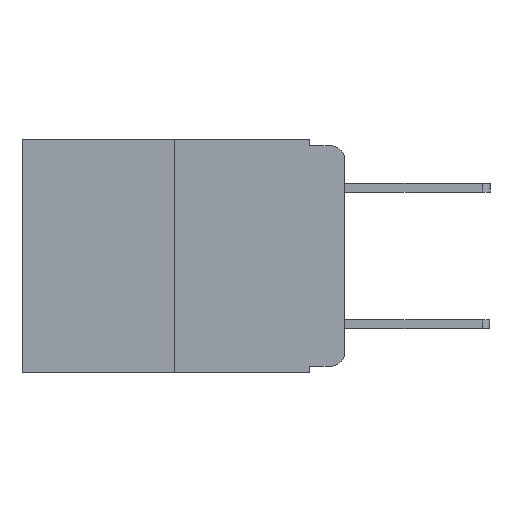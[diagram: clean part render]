
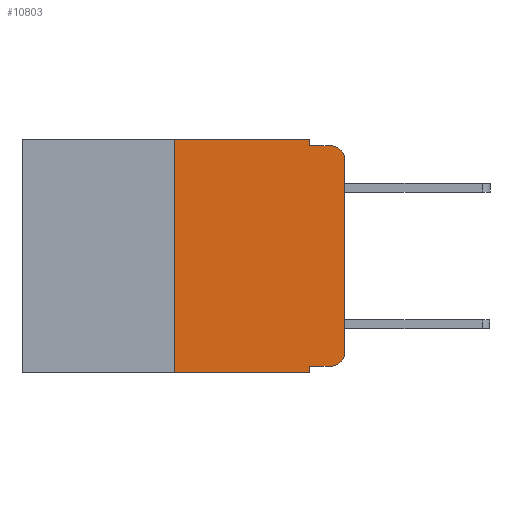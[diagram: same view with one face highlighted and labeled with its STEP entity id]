
A CAD part, left-side view. The second image highlights one B-rep face of the part: STEP entity #10803.
In plain terms, the highlighted planar face has unit normal (-1, 0, 0).
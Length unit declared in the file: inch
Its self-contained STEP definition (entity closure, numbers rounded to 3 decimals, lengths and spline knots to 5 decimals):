
#168 = LINE ( 'NONE', #14847, #4558 ) ;
#175 = LINE ( 'NONE', #13867, #18776 ) ;
#772 = ORIENTED_EDGE ( 'NONE', *, *, #3766, .T. ) ;
#1651 = ORIENTED_EDGE ( 'NONE', *, *, #4543, .F. ) ;
#1679 = VECTOR ( 'NONE', #12009, 39.37008 ) ;
#2320 = LINE ( 'NONE', #2339, #20710 ) ;
#2339 = CARTESIAN_POINT ( 'NONE',  ( 0., 0., 0. ) ) ;
#2484 = CARTESIAN_POINT ( 'NONE',  ( 0., 0.051, -0.333 ) ) ;
#2828 = EDGE_CURVE ( 'NONE', #6798, #6359, #2320, .T. ) ;
#2835 = CARTESIAN_POINT ( 'NONE',  ( 0., 0.02, -0.333 ) ) ;
#2984 = VERTEX_POINT ( 'NONE', #10625 ) ;
#3086 = VERTEX_POINT ( 'NONE', #10299 ) ;
#3766 = EDGE_CURVE ( 'NONE', #23074, #15496, #11955, .T. ) ;
#4369 = FACE_OUTER_BOUND ( 'NONE', #20748, .T. ) ;
#4543 = EDGE_CURVE ( 'NONE', #9731, #9596, #175, .T. ) ;
#4558 = VECTOR ( 'NONE', #9548, 39.37008 ) ;
#4666 = VECTOR ( 'NONE', #14319, 39.37008 ) ;
#4750 = AXIS2_PLACEMENT_3D ( 'NONE', #20246, #9752, #21972 ) ;
#4776 = LINE ( 'NONE', #7877, #17878 ) ;
#5048 = CARTESIAN_POINT ( 'NONE',  ( 0., 0.473, 0. ) ) ;
#5425 = ORIENTED_EDGE ( 'NONE', *, *, #19285, .F. ) ;
#5582 = CARTESIAN_POINT ( 'NONE',  ( 0., 0.25, 0. ) ) ;
#5977 = CARTESIAN_POINT ( 'NONE',  ( 0., 0.051, 0. ) ) ;
#6223 = EDGE_CURVE ( 'NONE', #23074, #15242, #4776, .T. ) ;
#6258 = EDGE_CURVE ( 'NONE', #2984, #15242, #22451, .T. ) ;
#6303 = ORIENTED_EDGE ( 'NONE', *, *, #10208, .T. ) ;
#6359 = VERTEX_POINT ( 'NONE', #14167 ) ;
#6413 = DIRECTION ( 'NONE',  ( 0., 0., -1. ) ) ;
#6798 = VERTEX_POINT ( 'NONE', #8709 ) ;
#6996 = EDGE_CURVE ( 'NONE', #3086, #23016, #12933, .T. ) ;
#7148 = AXIS2_PLACEMENT_3D ( 'NONE', #20542, #10077, #22284 ) ;
#7418 = ORIENTED_EDGE ( 'NONE', *, *, #2828, .T. ) ;
#7732 = DIRECTION ( 'NONE',  ( 0., -1., 0. ) ) ;
#7877 = CARTESIAN_POINT ( 'NONE',  ( 0., 0.051, 0. ) ) ;
#7896 = VECTOR ( 'NONE', #22745, 39.37008 ) ;
#8709 = CARTESIAN_POINT ( 'NONE',  ( 0., 0., -0.313 ) ) ;
#9112 = ORIENTED_EDGE ( 'NONE', *, *, #6996, .F. ) ;
#9129 = CARTESIAN_POINT ( 'NONE',  ( 0., 0.473, -0.343 ) ) ;
#9548 = DIRECTION ( 'NONE',  ( 0., 0., 1. ) ) ;
#9596 = VERTEX_POINT ( 'NONE', #5977 ) ;
#9731 = VERTEX_POINT ( 'NONE', #5582 ) ;
#9752 = DIRECTION ( 'NONE',  ( -1., 0., 0. ) ) ;
#10077 = DIRECTION ( 'NONE',  ( -1., 0., 0. ) ) ;
#10208 = EDGE_CURVE ( 'NONE', #15496, #6798, #22122, .T. ) ;
#10299 = CARTESIAN_POINT ( 'NONE',  ( 0., 0.051, -0.01 ) ) ;
#10394 = DIRECTION ( 'NONE',  ( 0., 0., 1. ) ) ;
#10507 = DIRECTION ( 'NONE',  ( 0., 0., -1. ) ) ;
#10625 = CARTESIAN_POINT ( 'NONE',  ( 0., 0.25, -0.343 ) ) ;
#10803 = ADVANCED_FACE ( 'NONE', ( #4369 ), #22634, .F. ) ;
#11955 = LINE ( 'NONE', #11986, #1679 ) ;
#11986 = CARTESIAN_POINT ( 'NONE',  ( 0., 0.051, -0.333 ) ) ;
#12009 = DIRECTION ( 'NONE',  ( 0., -1., 0. ) ) ;
#12540 = CARTESIAN_POINT ( 'NONE',  ( 0., 0.051, 0. ) ) ;
#12930 = CARTESIAN_POINT ( 'NONE',  ( 0., 0.051, -0.343 ) ) ;
#12933 = LINE ( 'NONE', #19776, #21065 ) ;
#13134 = LINE ( 'NONE', #12540, #4666 ) ;
#13308 = ORIENTED_EDGE ( 'NONE', *, *, #14182, .T. ) ;
#13439 = EDGE_CURVE ( 'NONE', #2984, #9731, #168, .T. ) ;
#13588 = ORIENTED_EDGE ( 'NONE', *, *, #6223, .F. ) ;
#13867 = CARTESIAN_POINT ( 'NONE',  ( 0., 0.473, 0. ) ) ;
#14167 = CARTESIAN_POINT ( 'NONE',  ( 0., 0., -0.03 ) ) ;
#14182 = EDGE_CURVE ( 'NONE', #6359, #23016, #14995, .T. ) ;
#14319 = DIRECTION ( 'NONE',  ( 0., 0., -1. ) ) ;
#14847 = CARTESIAN_POINT ( 'NONE',  ( 0., 0.25, 0. ) ) ;
#14995 = CIRCLE ( 'NONE', #4750, 0.02 ) ;
#15242 = VERTEX_POINT ( 'NONE', #12930 ) ;
#15496 = VERTEX_POINT ( 'NONE', #2835 ) ;
#15664 = AXIS2_PLACEMENT_3D ( 'NONE', #5048, #20970, #10507 ) ;
#16391 = DIRECTION ( 'NONE',  ( 0., -1., 0. ) ) ;
#16599 = ORIENTED_EDGE ( 'NONE', *, *, #13439, .F. ) ;
#17878 = VECTOR ( 'NONE', #6413, 39.37008 ) ;
#18776 = VECTOR ( 'NONE', #7732, 39.37008 ) ;
#19285 = EDGE_CURVE ( 'NONE', #9596, #3086, #13134, .T. ) ;
#19776 = CARTESIAN_POINT ( 'NONE',  ( 0., 0.051, -0.01 ) ) ;
#20104 = CARTESIAN_POINT ( 'NONE',  ( 0., 0.02, -0.01 ) ) ;
#20246 = CARTESIAN_POINT ( 'NONE',  ( 0., 0.02, -0.03 ) ) ;
#20542 = CARTESIAN_POINT ( 'NONE',  ( 0., 0.02, -0.313 ) ) ;
#20710 = VECTOR ( 'NONE', #10394, 39.37008 ) ;
#20748 = EDGE_LOOP ( 'NONE', ( #7418, #13308, #9112, #5425, #1651, #16599, #21720, #13588, #772, #6303 ) ) ;
#20970 = DIRECTION ( 'NONE',  ( 1., 0., 0. ) ) ;
#21065 = VECTOR ( 'NONE', #16391, 39.37008 ) ;
#21720 = ORIENTED_EDGE ( 'NONE', *, *, #6258, .T. ) ;
#21972 = DIRECTION ( 'NONE',  ( 0., 0., -1. ) ) ;
#22122 = CIRCLE ( 'NONE', #7148, 0.02 ) ;
#22284 = DIRECTION ( 'NONE',  ( 0., 0., -1. ) ) ;
#22451 = LINE ( 'NONE', #9129, #7896 ) ;
#22634 = PLANE ( 'NONE',  #15664 ) ;
#22745 = DIRECTION ( 'NONE',  ( 0., -1., 0. ) ) ;
#23016 = VERTEX_POINT ( 'NONE', #20104 ) ;
#23074 = VERTEX_POINT ( 'NONE', #2484 ) ;
